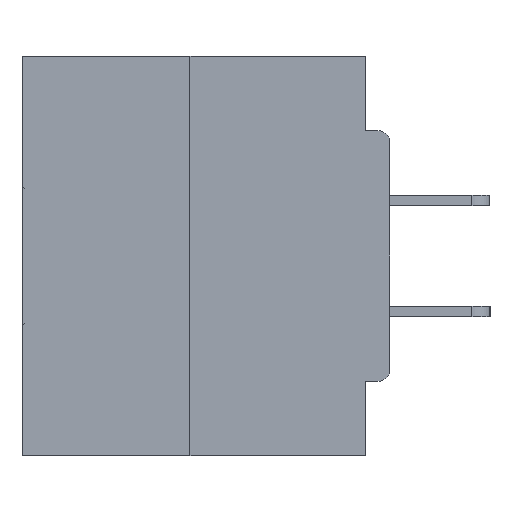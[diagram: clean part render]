
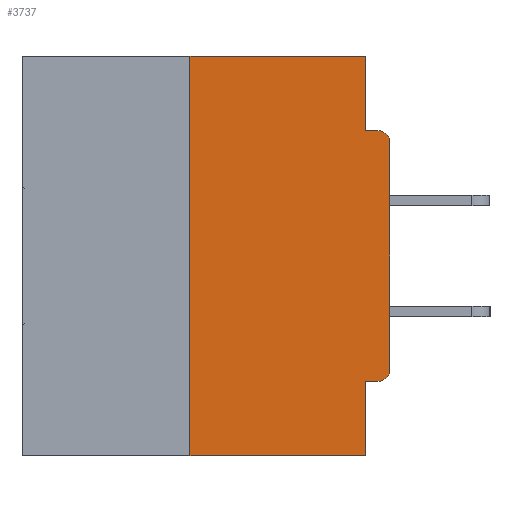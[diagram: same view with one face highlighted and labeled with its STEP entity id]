
A CAD part, left-side view. The second image highlights one B-rep face of the part: STEP entity #3737.
In plain terms, the highlighted planar face has unit normal (-1, 0, 0).
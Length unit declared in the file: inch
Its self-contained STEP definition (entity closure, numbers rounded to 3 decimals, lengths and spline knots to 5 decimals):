
#435 = VECTOR ( 'NONE', #5570, 39.37008 ) ;
#462 = ORIENTED_EDGE ( 'NONE', *, *, #18870, .T. ) ;
#705 = DIRECTION ( 'NONE',  ( 0., 0., -1. ) ) ;
#755 = DIRECTION ( 'NONE',  ( 0., 0., -1. ) ) ;
#783 = DIRECTION ( 'NONE',  ( -1., 0., 0. ) ) ;
#1666 = DIRECTION ( 'NONE',  ( 0., 0., -1. ) ) ;
#2231 = VERTEX_POINT ( 'NONE', #22087 ) ;
#2869 = ORIENTED_EDGE ( 'NONE', *, *, #31880, .F. ) ;
#3737 = ADVANCED_FACE ( 'NONE', ( #38501 ), #20229, .F. ) ;
#3910 = CARTESIAN_POINT ( 'NONE',  ( 0., 0., 0. ) ) ;
#4491 = CARTESIAN_POINT ( 'NONE',  ( 0., 0.25, -0.5 ) ) ;
#4763 = CARTESIAN_POINT ( 'NONE',  ( 0., 0.031, -0.5 ) ) ;
#4819 = EDGE_CURVE ( 'NONE', #18111, #20768, #15644, .T. ) ;
#4972 = CARTESIAN_POINT ( 'NONE',  ( 0., 0.031, 0. ) ) ;
#5264 = AXIS2_PLACEMENT_3D ( 'NONE', #32470, #22920, #755 ) ;
#5370 = CARTESIAN_POINT ( 'NONE',  ( 0., 0., -0.4065 ) ) ;
#5382 = ORIENTED_EDGE ( 'NONE', *, *, #40203, .F. ) ;
#5570 = DIRECTION ( 'NONE',  ( 0., 1., 0. ) ) ;
#5618 = CARTESIAN_POINT ( 'NONE',  ( 0., 0., -0.0935 ) ) ;
#6789 = DIRECTION ( 'NONE',  ( 0., 0., -1. ) ) ;
#7616 = VECTOR ( 'NONE', #8730, 39.37008 ) ;
#7659 = CARTESIAN_POINT ( 'NONE',  ( 0., 0.031, -0.4065 ) ) ;
#8730 = DIRECTION ( 'NONE',  ( 0., -1., 0. ) ) ;
#9173 = ORIENTED_EDGE ( 'NONE', *, *, #19193, .F. ) ;
#9529 = AXIS2_PLACEMENT_3D ( 'NONE', #39143, #783, #22955 ) ;
#10120 = CARTESIAN_POINT ( 'NONE',  ( 0., 0., -0.3915 ) ) ;
#10766 = EDGE_CURVE ( 'NONE', #2231, #39732, #20142, .T. ) ;
#10916 = EDGE_CURVE ( 'NONE', #18111, #14207, #39958, .T. ) ;
#11383 = ORIENTED_EDGE ( 'NONE', *, *, #10766, .T. ) ;
#11514 = VECTOR ( 'NONE', #23568, 39.37008 ) ;
#11945 = AXIS2_PLACEMENT_3D ( 'NONE', #13518, #16233, #705 ) ;
#12826 = DIRECTION ( 'NONE',  ( 0., 0., 1. ) ) ;
#13518 = CARTESIAN_POINT ( 'NONE',  ( 0., 0.015, -0.3915 ) ) ;
#13776 = CARTESIAN_POINT ( 'NONE',  ( 0., 0.015, -0.0935 ) ) ;
#14207 = VERTEX_POINT ( 'NONE', #35619 ) ;
#14488 = VECTOR ( 'NONE', #1666, 39.37008 ) ;
#14840 = CARTESIAN_POINT ( 'NONE',  ( 0., 0.46, -0.5 ) ) ;
#15168 = CARTESIAN_POINT ( 'NONE',  ( 0., 0.46, 0. ) ) ;
#15426 = VERTEX_POINT ( 'NONE', #4972 ) ;
#15644 = LINE ( 'NONE', #18758, #20028 ) ;
#16233 = DIRECTION ( 'NONE',  ( -1., 0., 0. ) ) ;
#16387 = ORIENTED_EDGE ( 'NONE', *, *, #10916, .T. ) ;
#17688 = CARTESIAN_POINT ( 'NONE',  ( 0., 0.25, 0. ) ) ;
#18081 = LINE ( 'NONE', #15168, #7616 ) ;
#18111 = VERTEX_POINT ( 'NONE', #4491 ) ;
#18710 = VECTOR ( 'NONE', #6789, 39.37008 ) ;
#18758 = CARTESIAN_POINT ( 'NONE',  ( 0., 0.25, 0. ) ) ;
#18870 = EDGE_CURVE ( 'NONE', #36407, #35186, #30537, .T. ) ;
#19064 = LINE ( 'NONE', #3910, #28905 ) ;
#19193 = EDGE_CURVE ( 'NONE', #32966, #39732, #28427, .T. ) ;
#20028 = VECTOR ( 'NONE', #34936, 39.37008 ) ;
#20142 = CIRCLE ( 'NONE', #9529, 0.015 ) ;
#20229 = PLANE ( 'NONE',  #5264 ) ;
#20768 = VERTEX_POINT ( 'NONE', #17688 ) ;
#21034 = EDGE_LOOP ( 'NONE', ( #28153, #21393, #16387, #5382, #36464, #462, #35546, #11383, #9173, #2869 ) ) ;
#21393 = ORIENTED_EDGE ( 'NONE', *, *, #4819, .F. ) ;
#22087 = CARTESIAN_POINT ( 'NONE',  ( 0., 0., -0.1085 ) ) ;
#22920 = DIRECTION ( 'NONE',  ( 1., 0., 0. ) ) ;
#22955 = DIRECTION ( 'NONE',  ( 0., 0., -1. ) ) ;
#23568 = DIRECTION ( 'NONE',  ( 0., -1., 0. ) ) ;
#24763 = EDGE_CURVE ( 'NONE', #35186, #2231, #19064, .T. ) ;
#25048 = LINE ( 'NONE', #5370, #435 ) ;
#26303 = VECTOR ( 'NONE', #34654, 39.37008 ) ;
#27501 = CARTESIAN_POINT ( 'NONE',  ( 0., 0.031, -0.0935 ) ) ;
#27621 = CARTESIAN_POINT ( 'NONE',  ( 0., 0.015, -0.4065 ) ) ;
#28153 = ORIENTED_EDGE ( 'NONE', *, *, #36360, .F. ) ;
#28427 = LINE ( 'NONE', #5618, #26303 ) ;
#28905 = VECTOR ( 'NONE', #12826, 39.37008 ) ;
#30537 = CIRCLE ( 'NONE', #11945, 0.015 ) ;
#31591 = VERTEX_POINT ( 'NONE', #7659 ) ;
#31745 = EDGE_CURVE ( 'NONE', #36407, #31591, #25048, .T. ) ;
#31880 = EDGE_CURVE ( 'NONE', #15426, #32966, #35222, .T. ) ;
#32311 = CARTESIAN_POINT ( 'NONE',  ( 0., 0.031, 0. ) ) ;
#32470 = CARTESIAN_POINT ( 'NONE',  ( 0., 0.46, 0. ) ) ;
#32966 = VERTEX_POINT ( 'NONE', #27501 ) ;
#33184 = LINE ( 'NONE', #4763, #14488 ) ;
#34654 = DIRECTION ( 'NONE',  ( 0., -1., 0. ) ) ;
#34936 = DIRECTION ( 'NONE',  ( 0., 0., 1. ) ) ;
#35186 = VERTEX_POINT ( 'NONE', #10120 ) ;
#35222 = LINE ( 'NONE', #32311, #18710 ) ;
#35546 = ORIENTED_EDGE ( 'NONE', *, *, #24763, .T. ) ;
#35619 = CARTESIAN_POINT ( 'NONE',  ( 0., 0.031, -0.5 ) ) ;
#36360 = EDGE_CURVE ( 'NONE', #20768, #15426, #18081, .T. ) ;
#36407 = VERTEX_POINT ( 'NONE', #27621 ) ;
#36464 = ORIENTED_EDGE ( 'NONE', *, *, #31745, .F. ) ;
#38501 = FACE_OUTER_BOUND ( 'NONE', #21034, .T. ) ;
#39143 = CARTESIAN_POINT ( 'NONE',  ( 0., 0.015, -0.1085 ) ) ;
#39732 = VERTEX_POINT ( 'NONE', #13776 ) ;
#39958 = LINE ( 'NONE', #14840, #11514 ) ;
#40203 = EDGE_CURVE ( 'NONE', #31591, #14207, #33184, .T. ) ;
